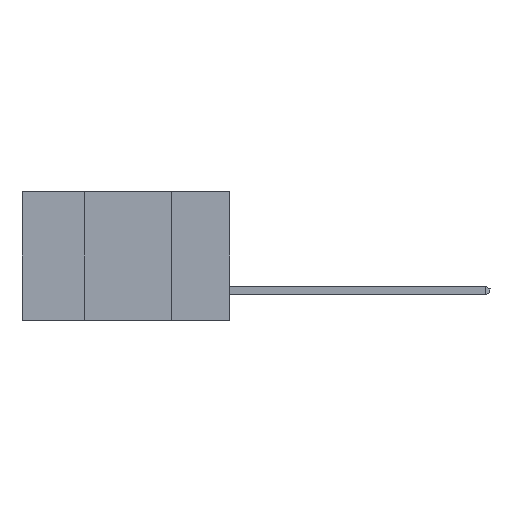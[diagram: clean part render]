
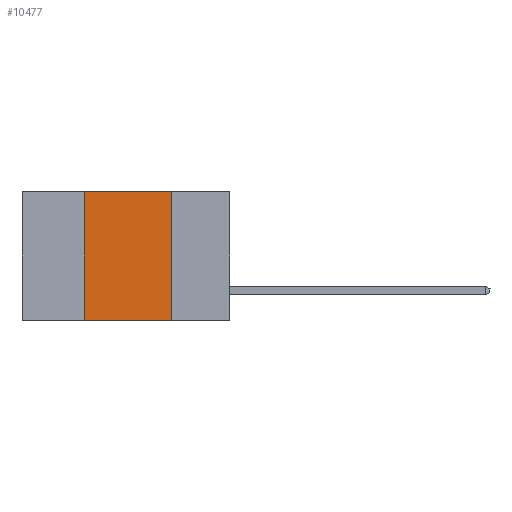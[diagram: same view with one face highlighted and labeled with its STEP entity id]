
A CAD part, left-side view. The second image highlights one B-rep face of the part: STEP entity #10477.
In plain terms, the highlighted planar face has unit normal (-1, 0, 0).
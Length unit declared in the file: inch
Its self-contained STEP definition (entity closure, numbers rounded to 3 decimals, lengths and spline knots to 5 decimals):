
#82 = EDGE_CURVE ( 'NONE', #7191, #12944, #15664, .T. ) ;
#418 = EDGE_CURVE ( 'NONE', #1747, #11718, #4803, .T. ) ;
#1244 = ORIENTED_EDGE ( 'NONE', *, *, #15278, .T. ) ;
#1344 = CARTESIAN_POINT ( 'NONE',  ( 0., 0.42, -0.37 ) ) ;
#1420 = VECTOR ( 'NONE', #6469, 39.37008 ) ;
#1710 = ORIENTED_EDGE ( 'NONE', *, *, #7488, .F. ) ;
#1747 = VERTEX_POINT ( 'NONE', #12626 ) ;
#2157 = DIRECTION ( 'NONE',  ( 0., 0., -1. ) ) ;
#2257 = VECTOR ( 'NONE', #3509, 39.37008 ) ;
#3509 = DIRECTION ( 'NONE',  ( 0., 0., -1. ) ) ;
#3522 = CARTESIAN_POINT ( 'NONE',  ( 0., 0.6, -0.37 ) ) ;
#4370 = CARTESIAN_POINT ( 'NONE',  ( 0., 0.42, 0. ) ) ;
#4803 = LINE ( 'NONE', #12549, #2257 ) ;
#5976 = PLANE ( 'NONE',  #13849 ) ;
#6262 = CARTESIAN_POINT ( 'NONE',  ( 0., 0.42, -0.37 ) ) ;
#6382 = LINE ( 'NONE', #3522, #12573 ) ;
#6469 = DIRECTION ( 'NONE',  ( 0., 0., 1. ) ) ;
#7191 = VERTEX_POINT ( 'NONE', #6262 ) ;
#7315 = EDGE_LOOP ( 'NONE', ( #14110, #1710, #7479, #1244 ) ) ;
#7479 = ORIENTED_EDGE ( 'NONE', *, *, #82, .F. ) ;
#7488 = EDGE_CURVE ( 'NONE', #12944, #1747, #13638, .T. ) ;
#8530 = CARTESIAN_POINT ( 'NONE',  ( 0., 0.17, -0.37 ) ) ;
#10477 = ADVANCED_FACE ( 'NONE', ( #16464 ), #5976, .F. ) ;
#11117 = CARTESIAN_POINT ( 'NONE',  ( 0., 0.6, 0. ) ) ;
#11534 = CARTESIAN_POINT ( 'NONE',  ( 0., 0.6, 0. ) ) ;
#11682 = DIRECTION ( 'NONE',  ( 0., -1., 0. ) ) ;
#11718 = VERTEX_POINT ( 'NONE', #8530 ) ;
#12549 = CARTESIAN_POINT ( 'NONE',  ( 0., 0.17, -0.37 ) ) ;
#12573 = VECTOR ( 'NONE', #11682, 39.37008 ) ;
#12626 = CARTESIAN_POINT ( 'NONE',  ( 0., 0.17, 0. ) ) ;
#12841 = DIRECTION ( 'NONE',  ( 1., 0., 0. ) ) ;
#12944 = VERTEX_POINT ( 'NONE', #4370 ) ;
#13261 = VECTOR ( 'NONE', #15019, 39.37008 ) ;
#13638 = LINE ( 'NONE', #11117, #13261 ) ;
#13849 = AXIS2_PLACEMENT_3D ( 'NONE', #11534, #12841, #2157 ) ;
#14110 = ORIENTED_EDGE ( 'NONE', *, *, #418, .F. ) ;
#15019 = DIRECTION ( 'NONE',  ( 0., -1., 0. ) ) ;
#15278 = EDGE_CURVE ( 'NONE', #7191, #11718, #6382, .T. ) ;
#15664 = LINE ( 'NONE', #1344, #1420 ) ;
#16464 = FACE_OUTER_BOUND ( 'NONE', #7315, .T. ) ;
